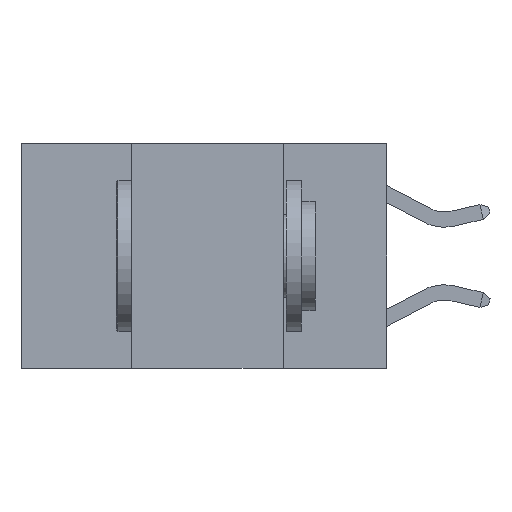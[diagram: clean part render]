
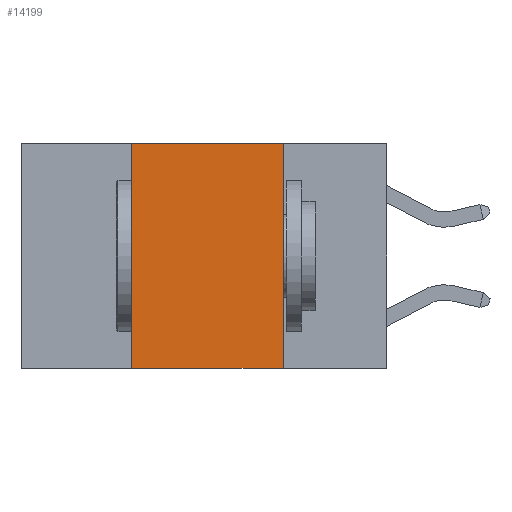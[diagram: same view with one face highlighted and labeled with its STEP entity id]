
A CAD part, left-side view. The second image highlights one B-rep face of the part: STEP entity #14199.
In plain terms, the highlighted planar face has unit normal (-1, 0, 0).
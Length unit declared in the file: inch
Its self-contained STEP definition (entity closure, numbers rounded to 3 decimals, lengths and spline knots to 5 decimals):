
#2444 = DIRECTION ( 'NONE',  ( 1., 0., 0. ) ) ;
#3986 = LINE ( 'NONE', #6087, #27784 ) ;
#4294 = VECTOR ( 'NONE', #6821, 39.37008 ) ;
#5604 = ORIENTED_EDGE ( 'NONE', *, *, #16884, .F. ) ;
#5688 = EDGE_CURVE ( 'NONE', #10338, #25953, #15897, .T. ) ;
#6087 = CARTESIAN_POINT ( 'NONE',  ( 0., 0.42, 0. ) ) ;
#6821 = DIRECTION ( 'NONE',  ( 0., -1., 0. ) ) ;
#7087 = EDGE_CURVE ( 'NONE', #20096, #15957, #21764, .T. ) ;
#8034 = ORIENTED_EDGE ( 'NONE', *, *, #7087, .F. ) ;
#9500 = ORIENTED_EDGE ( 'NONE', *, *, #16481, .F. ) ;
#10338 = VERTEX_POINT ( 'NONE', #25132 ) ;
#11099 = DIRECTION ( 'NONE',  ( 0., -1., 0. ) ) ;
#12562 = DIRECTION ( 'NONE',  ( 0., 0., 1. ) ) ;
#12706 = CARTESIAN_POINT ( 'NONE',  ( 0., 0.42, 0. ) ) ;
#13283 = FACE_OUTER_BOUND ( 'NONE', #15119, .T. ) ;
#13482 = CARTESIAN_POINT ( 'NONE',  ( 0., 0.6, 0. ) ) ;
#14199 = ADVANCED_FACE ( 'NONE', ( #13283 ), #17771, .F. ) ;
#14999 = CARTESIAN_POINT ( 'NONE',  ( 0., 0.17, 0. ) ) ;
#15119 = EDGE_LOOP ( 'NONE', ( #9500, #8034, #5604, #18230 ) ) ;
#15250 = LINE ( 'NONE', #21425, #18735 ) ;
#15897 = LINE ( 'NONE', #20251, #4294 ) ;
#15957 = VERTEX_POINT ( 'NONE', #14999 ) ;
#16481 = EDGE_CURVE ( 'NONE', #15957, #25953, #15250, .T. ) ;
#16884 = EDGE_CURVE ( 'NONE', #10338, #20096, #3986, .T. ) ;
#17771 = PLANE ( 'NONE',  #21421 ) ;
#18230 = ORIENTED_EDGE ( 'NONE', *, *, #5688, .T. ) ;
#18699 = VECTOR ( 'NONE', #11099, 39.37008 ) ;
#18735 = VECTOR ( 'NONE', #27802, 39.37008 ) ;
#20096 = VERTEX_POINT ( 'NONE', #12706 ) ;
#20251 = CARTESIAN_POINT ( 'NONE',  ( 0., 0.6, -0.37 ) ) ;
#21421 = AXIS2_PLACEMENT_3D ( 'NONE', #23978, #2444, #24121 ) ;
#21425 = CARTESIAN_POINT ( 'NONE',  ( 0., 0.17, 0. ) ) ;
#21764 = LINE ( 'NONE', #13482, #18699 ) ;
#23978 = CARTESIAN_POINT ( 'NONE',  ( 0., 0.6, 0. ) ) ;
#24121 = DIRECTION ( 'NONE',  ( 0., 0., -1. ) ) ;
#25132 = CARTESIAN_POINT ( 'NONE',  ( 0., 0.42, -0.37 ) ) ;
#25953 = VERTEX_POINT ( 'NONE', #27540 ) ;
#27540 = CARTESIAN_POINT ( 'NONE',  ( 0., 0.17, -0.37 ) ) ;
#27784 = VECTOR ( 'NONE', #12562, 39.37008 ) ;
#27802 = DIRECTION ( 'NONE',  ( 0., 0., -1. ) ) ;
